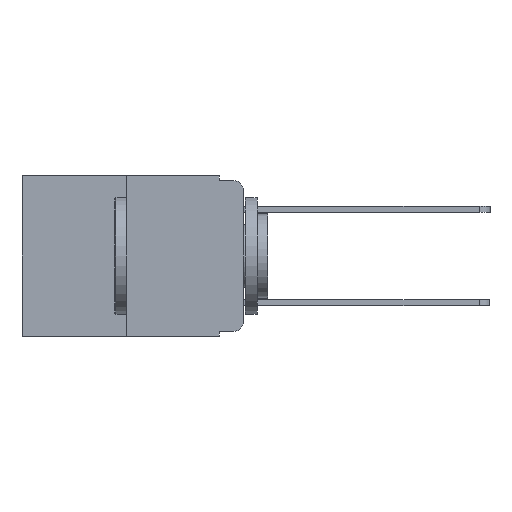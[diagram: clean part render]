
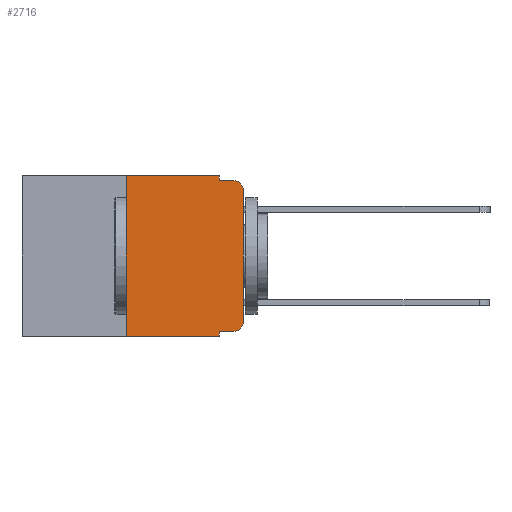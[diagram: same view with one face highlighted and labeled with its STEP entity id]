
A CAD part, left-side view. The second image highlights one B-rep face of the part: STEP entity #2716.
In plain terms, the highlighted planar face has unit normal (-1, 0, 0).
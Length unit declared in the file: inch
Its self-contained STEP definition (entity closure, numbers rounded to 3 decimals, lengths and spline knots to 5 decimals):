
#25 = EDGE_LOOP ( 'NONE', ( #594, #3595, #6057, #3032, #7479, #9873, #10120, #10628, #134, #7862 ) ) ;
#84 = EDGE_CURVE ( 'NONE', #3014, #3280, #8986, .T. ) ;
#132 = LINE ( 'NONE', #7374, #9247 ) ;
#134 = ORIENTED_EDGE ( 'NONE', *, *, #9727, .T. ) ;
#423 = VECTOR ( 'NONE', #3214, 39.37008 ) ;
#450 = CARTESIAN_POINT ( 'NONE',  ( 0., 0.051, -0.01 ) ) ;
#594 = ORIENTED_EDGE ( 'NONE', *, *, #5141, .T. ) ;
#766 = CARTESIAN_POINT ( 'NONE',  ( 0., 0.25, -0.343 ) ) ;
#906 = VERTEX_POINT ( 'NONE', #9635 ) ;
#1244 = FACE_OUTER_BOUND ( 'NONE', #25, .T. ) ;
#1743 = VERTEX_POINT ( 'NONE', #2272 ) ;
#1821 = CARTESIAN_POINT ( 'NONE',  ( 0., 0.473, -0.343 ) ) ;
#1855 = DIRECTION ( 'NONE',  ( -1., 0., 0. ) ) ;
#2075 = CARTESIAN_POINT ( 'NONE',  ( 0., 0.02, -0.01 ) ) ;
#2215 = EDGE_CURVE ( 'NONE', #3280, #5767, #7551, .T. ) ;
#2272 = CARTESIAN_POINT ( 'NONE',  ( 0., 0.051, -0.343 ) ) ;
#2537 = CARTESIAN_POINT ( 'NONE',  ( 0., 0., -0.313 ) ) ;
#2716 = ADVANCED_FACE ( 'NONE', ( #1244 ), #5992, .F. ) ;
#3014 = VERTEX_POINT ( 'NONE', #6725 ) ;
#3032 = ORIENTED_EDGE ( 'NONE', *, *, #84, .F. ) ;
#3214 = DIRECTION ( 'NONE',  ( 0., -1., 0. ) ) ;
#3280 = VERTEX_POINT ( 'NONE', #5530 ) ;
#3453 = DIRECTION ( 'NONE',  ( 0., 0., 1. ) ) ;
#3467 = EDGE_CURVE ( 'NONE', #6203, #5767, #9023, .T. ) ;
#3595 = ORIENTED_EDGE ( 'NONE', *, *, #3467, .T. ) ;
#3771 = VERTEX_POINT ( 'NONE', #2537 ) ;
#3953 = VECTOR ( 'NONE', #5682, 39.37008 ) ;
#4051 = EDGE_CURVE ( 'NONE', #5544, #1743, #4133, .T. ) ;
#4133 = LINE ( 'NONE', #1821, #6325 ) ;
#4385 = CIRCLE ( 'NONE', #8867, 0.02 ) ;
#4464 = VECTOR ( 'NONE', #3453, 39.37008 ) ;
#4561 = DIRECTION ( 'NONE',  ( 0., -1., 0. ) ) ;
#4618 = VECTOR ( 'NONE', #6364, 39.37008 ) ;
#4722 = LINE ( 'NONE', #5953, #4464 ) ;
#4912 = DIRECTION ( 'NONE',  ( 0., 0., 1. ) ) ;
#5141 = EDGE_CURVE ( 'NONE', #3771, #6203, #132, .T. ) ;
#5314 = CARTESIAN_POINT ( 'NONE',  ( 0., 0.051, 0. ) ) ;
#5530 = CARTESIAN_POINT ( 'NONE',  ( 0., 0.051, -0.01 ) ) ;
#5544 = VERTEX_POINT ( 'NONE', #766 ) ;
#5583 = CARTESIAN_POINT ( 'NONE',  ( 0., 0.02, -0.03 ) ) ;
#5682 = DIRECTION ( 'NONE',  ( 0., 0., -1. ) ) ;
#5767 = VERTEX_POINT ( 'NONE', #2075 ) ;
#5822 = CARTESIAN_POINT ( 'NONE',  ( 0., 0.25, 0. ) ) ;
#5899 = VECTOR ( 'NONE', #7537, 39.37008 ) ;
#5953 = CARTESIAN_POINT ( 'NONE',  ( 0., 0.25, 0. ) ) ;
#5990 = DIRECTION ( 'NONE',  ( 1., 0., 0. ) ) ;
#5992 = PLANE ( 'NONE',  #7695 ) ;
#6057 = ORIENTED_EDGE ( 'NONE', *, *, #2215, .F. ) ;
#6086 = CARTESIAN_POINT ( 'NONE',  ( 0., 0.473, 0. ) ) ;
#6148 = LINE ( 'NONE', #8159, #3953 ) ;
#6187 = DIRECTION ( 'NONE',  ( 0., -1., 0. ) ) ;
#6203 = VERTEX_POINT ( 'NONE', #8448 ) ;
#6325 = VECTOR ( 'NONE', #4561, 39.37008 ) ;
#6364 = DIRECTION ( 'NONE',  ( 0., 0., -1. ) ) ;
#6410 = DIRECTION ( 'NONE',  ( 0., 0., -1. ) ) ;
#6725 = CARTESIAN_POINT ( 'NONE',  ( 0., 0.051, 0. ) ) ;
#7055 = CARTESIAN_POINT ( 'NONE',  ( 0., 0.02, -0.313 ) ) ;
#7374 = CARTESIAN_POINT ( 'NONE',  ( 0., 0., 0. ) ) ;
#7479 = ORIENTED_EDGE ( 'NONE', *, *, #9226, .F. ) ;
#7537 = DIRECTION ( 'NONE',  ( 0., -1., 0. ) ) ;
#7551 = LINE ( 'NONE', #450, #423 ) ;
#7695 = AXIS2_PLACEMENT_3D ( 'NONE', #6086, #5990, #8275 ) ;
#7820 = CARTESIAN_POINT ( 'NONE',  ( 0., 0.473, 0. ) ) ;
#7862 = ORIENTED_EDGE ( 'NONE', *, *, #8630, .T. ) ;
#7871 = DIRECTION ( 'NONE',  ( 0., 0., -1. ) ) ;
#8085 = LINE ( 'NONE', #9931, #5899 ) ;
#8095 = VECTOR ( 'NONE', #6187, 39.37008 ) ;
#8159 = CARTESIAN_POINT ( 'NONE',  ( 0., 0.051, 0. ) ) ;
#8275 = DIRECTION ( 'NONE',  ( 0., 0., -1. ) ) ;
#8345 = LINE ( 'NONE', #7820, #8095 ) ;
#8448 = CARTESIAN_POINT ( 'NONE',  ( 0., 0., -0.03 ) ) ;
#8630 = EDGE_CURVE ( 'NONE', #906, #3771, #4385, .T. ) ;
#8867 = AXIS2_PLACEMENT_3D ( 'NONE', #7055, #1855, #7871 ) ;
#8986 = LINE ( 'NONE', #5314, #4618 ) ;
#9023 = CIRCLE ( 'NONE', #11013, 0.02 ) ;
#9226 = EDGE_CURVE ( 'NONE', #10405, #3014, #8345, .T. ) ;
#9247 = VECTOR ( 'NONE', #4912, 39.37008 ) ;
#9635 = CARTESIAN_POINT ( 'NONE',  ( 0., 0.02, -0.333 ) ) ;
#9727 = EDGE_CURVE ( 'NONE', #10640, #906, #8085, .T. ) ;
#9873 = ORIENTED_EDGE ( 'NONE', *, *, #10817, .F. ) ;
#9883 = CARTESIAN_POINT ( 'NONE',  ( 0., 0.051, -0.333 ) ) ;
#9931 = CARTESIAN_POINT ( 'NONE',  ( 0., 0.051, -0.333 ) ) ;
#10120 = ORIENTED_EDGE ( 'NONE', *, *, #4051, .T. ) ;
#10260 = EDGE_CURVE ( 'NONE', #10640, #1743, #6148, .T. ) ;
#10405 = VERTEX_POINT ( 'NONE', #5822 ) ;
#10628 = ORIENTED_EDGE ( 'NONE', *, *, #10260, .F. ) ;
#10640 = VERTEX_POINT ( 'NONE', #9883 ) ;
#10817 = EDGE_CURVE ( 'NONE', #5544, #10405, #4722, .T. ) ;
#11013 = AXIS2_PLACEMENT_3D ( 'NONE', #5583, #11264, #6410 ) ;
#11264 = DIRECTION ( 'NONE',  ( -1., 0., 0. ) ) ;
